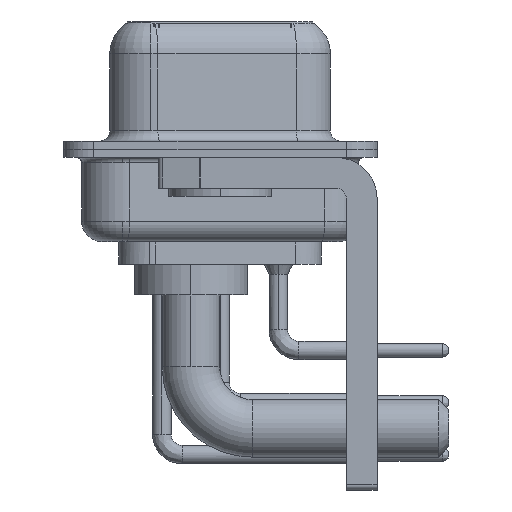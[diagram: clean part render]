
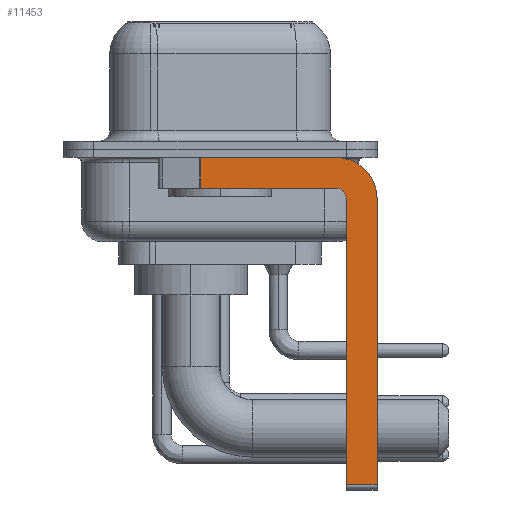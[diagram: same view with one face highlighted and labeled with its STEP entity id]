
A CAD part, left-side view. The second image highlights one B-rep face of the part: STEP entity #11453.
In plain terms, the highlighted planar face has unit normal (-1, 0, 0).
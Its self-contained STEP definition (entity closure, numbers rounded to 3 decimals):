
#386 = CARTESIAN_POINT ( 'NONE',  ( -2.9, 0.978, -1.9 ) ) ;
#577 = CARTESIAN_POINT ( 'NONE',  ( -2.9, -6.15, -16.35 ) ) ;
#1138 = VECTOR ( 'NONE', #13883, 1000. ) ;
#1366 = EDGE_CURVE ( 'NONE', #19854, #22988, #29176, .T. ) ;
#1415 = FACE_OUTER_BOUND ( 'NONE', #22216, .T. ) ;
#1855 = ORIENTED_EDGE ( 'NONE', *, *, #9273, .T. ) ;
#2681 = VERTEX_POINT ( 'NONE', #32689 ) ;
#2713 = ORIENTED_EDGE ( 'NONE', *, *, #15367, .F. ) ;
#2723 = VERTEX_POINT ( 'NONE', #7450 ) ;
#3326 = EDGE_CURVE ( 'NONE', #2681, #2723, #6613, .T. ) ;
#3620 = CARTESIAN_POINT ( 'NONE',  ( -2.9, -5.65, -2.4 ) ) ;
#5164 = DIRECTION ( 'NONE',  ( 0., -1., 0. ) ) ;
#5411 = ORIENTED_EDGE ( 'NONE', *, *, #27646, .F. ) ;
#6307 = DIRECTION ( 'NONE',  ( 1., 0., 0. ) ) ;
#6613 = CIRCLE ( 'NONE', #27558, 2. ) ;
#7095 = LINE ( 'NONE', #14523, #13318 ) ;
#7450 = CARTESIAN_POINT ( 'NONE',  ( -2.9, -7.65, -2.4 ) ) ;
#9273 = EDGE_CURVE ( 'NONE', #16272, #13146, #7095, .T. ) ;
#9302 = DIRECTION ( 'NONE',  ( 0., 0., 1. ) ) ;
#10215 = CARTESIAN_POINT ( 'NONE',  ( -2.9, 3., -0.4 ) ) ;
#10512 = ORIENTED_EDGE ( 'NONE', *, *, #15053, .F. ) ;
#11453 = ADVANCED_FACE ( 'NONE', ( #1415 ), #31898, .F. ) ;
#11473 = CARTESIAN_POINT ( 'NONE',  ( -2.9, -6.15, -16.6 ) ) ;
#11819 = LINE ( 'NONE', #14363, #21117 ) ;
#12376 = VERTEX_POINT ( 'NONE', #32097 ) ;
#13146 = VERTEX_POINT ( 'NONE', #386 ) ;
#13318 = VECTOR ( 'NONE', #24763, 1000. ) ;
#13725 = CARTESIAN_POINT ( 'NONE',  ( -2.9, -5.65, -16.35 ) ) ;
#13883 = DIRECTION ( 'NONE',  ( 0., -1., 0. ) ) ;
#14363 = CARTESIAN_POINT ( 'NONE',  ( -2.9, -5.65, -1.9 ) ) ;
#14523 = CARTESIAN_POINT ( 'NONE',  ( -2.9, 0.978, -1.9 ) ) ;
#15053 = EDGE_CURVE ( 'NONE', #19854, #21053, #26765, .T. ) ;
#15367 = EDGE_CURVE ( 'NONE', #2723, #22988, #17479, .T. ) ;
#16272 = VERTEX_POINT ( 'NONE', #25488 ) ;
#16576 = DIRECTION ( 'NONE',  ( 0., 0., -1. ) ) ;
#17278 = EDGE_CURVE ( 'NONE', #16272, #2681, #33263, .T. ) ;
#17479 = LINE ( 'NONE', #23027, #22194 ) ;
#18000 = DIRECTION ( 'NONE',  ( 1., 0., 0. ) ) ;
#19659 = CARTESIAN_POINT ( 'NONE',  ( -2.9, -6.15, -2.4 ) ) ;
#19854 = VERTEX_POINT ( 'NONE', #577 ) ;
#20591 = CARTESIAN_POINT ( 'NONE',  ( -2.9, -7.65, -16.35 ) ) ;
#21053 = VERTEX_POINT ( 'NONE', #19659 ) ;
#21117 = VECTOR ( 'NONE', #24595, 1000. ) ;
#21904 = CARTESIAN_POINT ( 'NONE',  ( -2.9, -5.65, -2.4 ) ) ;
#22194 = VECTOR ( 'NONE', #28081, 1000. ) ;
#22216 = EDGE_LOOP ( 'NONE', ( #23871, #1855, #5411, #25660, #10512, #23927, #2713, #26057 ) ) ;
#22768 = VECTOR ( 'NONE', #5164, 1000. ) ;
#22988 = VERTEX_POINT ( 'NONE', #20591 ) ;
#23027 = CARTESIAN_POINT ( 'NONE',  ( -2.9, -7.65, -2.4 ) ) ;
#23046 = CARTESIAN_POINT ( 'NONE',  ( -2.9, -5.65, -2.4 ) ) ;
#23327 = EDGE_CURVE ( 'NONE', #21053, #12376, #28983, .T. ) ;
#23871 = ORIENTED_EDGE ( 'NONE', *, *, #17278, .F. ) ;
#23913 = DIRECTION ( 'NONE',  ( 0., 0., 1. ) ) ;
#23927 = ORIENTED_EDGE ( 'NONE', *, *, #1366, .T. ) ;
#24595 = DIRECTION ( 'NONE',  ( 0., 1., 0. ) ) ;
#24763 = DIRECTION ( 'NONE',  ( 0., 0., -1. ) ) ;
#24841 = VECTOR ( 'NONE', #23913, 1000. ) ;
#25488 = CARTESIAN_POINT ( 'NONE',  ( -2.9, 0.978, -0.4 ) ) ;
#25660 = ORIENTED_EDGE ( 'NONE', *, *, #23327, .F. ) ;
#26057 = ORIENTED_EDGE ( 'NONE', *, *, #3326, .F. ) ;
#26765 = LINE ( 'NONE', #11473, #24841 ) ;
#27558 = AXIS2_PLACEMENT_3D ( 'NONE', #23046, #18000, #28265 ) ;
#27646 = EDGE_CURVE ( 'NONE', #12376, #13146, #11819, .T. ) ;
#27850 = AXIS2_PLACEMENT_3D ( 'NONE', #3620, #6307, #16576 ) ;
#28081 = DIRECTION ( 'NONE',  ( 0., 0., -1. ) ) ;
#28265 = DIRECTION ( 'NONE',  ( 0., 0., -1. ) ) ;
#28983 = CIRCLE ( 'NONE', #30590, 0.5 ) ;
#29176 = LINE ( 'NONE', #13725, #1138 ) ;
#29486 = DIRECTION ( 'NONE',  ( -1., 0., 0. ) ) ;
#30590 = AXIS2_PLACEMENT_3D ( 'NONE', #21904, #29486, #9302 ) ;
#31898 = PLANE ( 'NONE',  #27850 ) ;
#32097 = CARTESIAN_POINT ( 'NONE',  ( -2.9, -5.65, -1.9 ) ) ;
#32689 = CARTESIAN_POINT ( 'NONE',  ( -2.9, -5.65, -0.4 ) ) ;
#33263 = LINE ( 'NONE', #10215, #22768 ) ;
